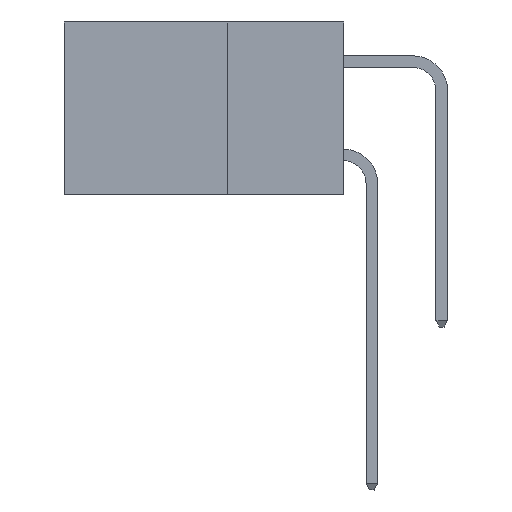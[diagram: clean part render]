
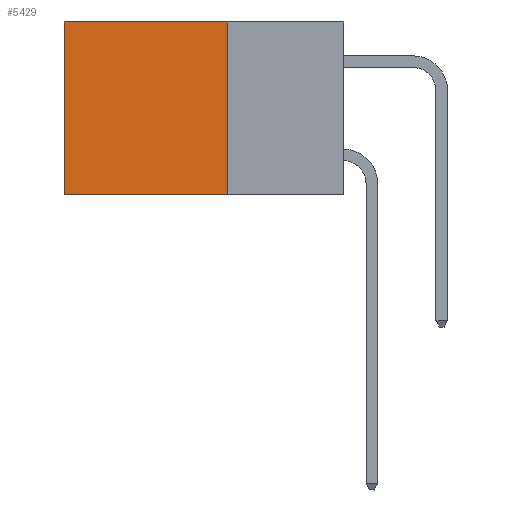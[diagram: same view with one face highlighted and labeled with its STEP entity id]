
A CAD part, left-side view. The second image highlights one B-rep face of the part: STEP entity #5429.
In plain terms, the highlighted planar face has unit normal (-1, 0, 0).
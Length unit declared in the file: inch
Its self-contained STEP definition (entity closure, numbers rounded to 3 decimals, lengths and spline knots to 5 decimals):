
#371 = VERTEX_POINT ( 'NONE', #10447 ) ;
#1659 = CARTESIAN_POINT ( 'NONE',  ( 0.298, 0.25, -0.37 ) ) ;
#3124 = CARTESIAN_POINT ( 'NONE',  ( 0.298, 0.6, -0.37 ) ) ;
#3577 = LINE ( 'NONE', #10415, #10181 ) ;
#3753 = VECTOR ( 'NONE', #9551, 39.37008 ) ;
#3808 = VECTOR ( 'NONE', #16049, 39.37008 ) ;
#4128 = ORIENTED_EDGE ( 'NONE', *, *, #10057, .F. ) ;
#4213 = LINE ( 'NONE', #1659, #3808 ) ;
#4264 = VERTEX_POINT ( 'NONE', #3124 ) ;
#4371 = CARTESIAN_POINT ( 'NONE',  ( 0.298, 0.6, 0. ) ) ;
#4744 = VERTEX_POINT ( 'NONE', #6079 ) ;
#4843 = EDGE_CURVE ( 'NONE', #7770, #4264, #11216, .T. ) ;
#5421 = PLANE ( 'NONE',  #7438 ) ;
#5429 = ADVANCED_FACE ( 'NONE', ( #9516 ), #5421, .F. ) ;
#6004 = CARTESIAN_POINT ( 'NONE',  ( 0.298, 0.25, 0. ) ) ;
#6079 = CARTESIAN_POINT ( 'NONE',  ( 0.298, 0.25, -0.37 ) ) ;
#6436 = ORIENTED_EDGE ( 'NONE', *, *, #4843, .T. ) ;
#7438 = AXIS2_PLACEMENT_3D ( 'NONE', #6004, #9092, #7777 ) ;
#7770 = VERTEX_POINT ( 'NONE', #4371 ) ;
#7777 = DIRECTION ( 'NONE',  ( 0., 0., -1. ) ) ;
#8006 = ORIENTED_EDGE ( 'NONE', *, *, #16118, .F. ) ;
#8732 = EDGE_CURVE ( 'NONE', #371, #7770, #14347, .T. ) ;
#9092 = DIRECTION ( 'NONE',  ( 1., 0., 0. ) ) ;
#9516 = FACE_OUTER_BOUND ( 'NONE', #11728, .T. ) ;
#9551 = DIRECTION ( 'NONE',  ( 0., 0., -1. ) ) ;
#10001 = VECTOR ( 'NONE', #16636, 39.37008 ) ;
#10057 = EDGE_CURVE ( 'NONE', #371, #4744, #3577, .T. ) ;
#10181 = VECTOR ( 'NONE', #12825, 39.37008 ) ;
#10415 = CARTESIAN_POINT ( 'NONE',  ( 0.298, 0.25, 0. ) ) ;
#10447 = CARTESIAN_POINT ( 'NONE',  ( 0.298, 0.25, 0. ) ) ;
#11216 = LINE ( 'NONE', #13750, #3753 ) ;
#11728 = EDGE_LOOP ( 'NONE', ( #6436, #8006, #4128, #13964 ) ) ;
#12125 = CARTESIAN_POINT ( 'NONE',  ( 0.298, 0.25, 0. ) ) ;
#12825 = DIRECTION ( 'NONE',  ( 0., 0., -1. ) ) ;
#13750 = CARTESIAN_POINT ( 'NONE',  ( 0.298, 0.6, 0. ) ) ;
#13964 = ORIENTED_EDGE ( 'NONE', *, *, #8732, .T. ) ;
#14347 = LINE ( 'NONE', #12125, #10001 ) ;
#16049 = DIRECTION ( 'NONE',  ( 0., 1., 0. ) ) ;
#16118 = EDGE_CURVE ( 'NONE', #4744, #4264, #4213, .T. ) ;
#16636 = DIRECTION ( 'NONE',  ( 0., 1., 0. ) ) ;
